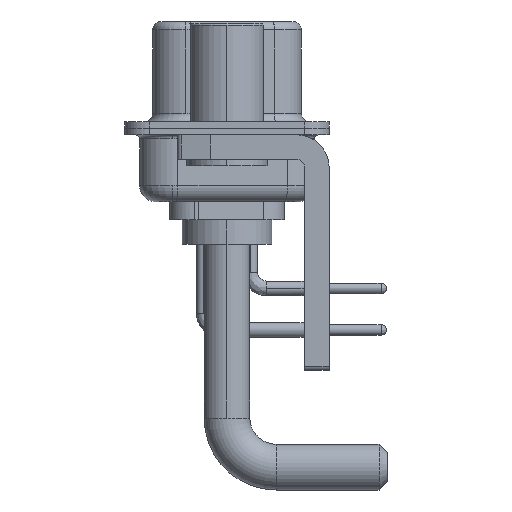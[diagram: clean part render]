
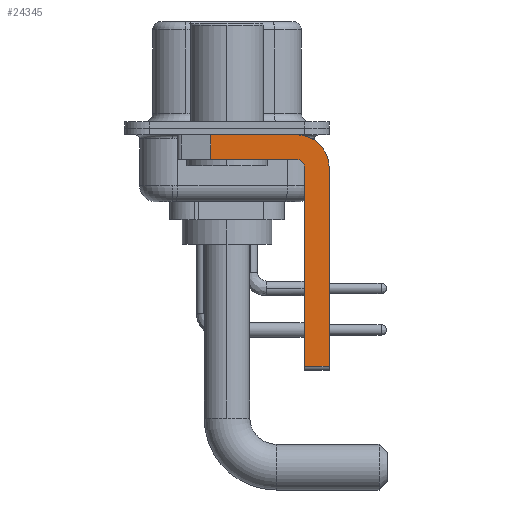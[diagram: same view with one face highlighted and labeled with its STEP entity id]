
A CAD part, left-side view. The second image highlights one B-rep face of the part: STEP entity #24345.
In plain terms, the highlighted planar face has unit normal (-1, 0, 0).
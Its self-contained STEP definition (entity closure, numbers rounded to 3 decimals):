
#410 = EDGE_CURVE ( 'NONE', #25710, #27441, #6920, .T. ) ;
#565 = DIRECTION ( 'NONE',  ( 0., -1., 0. ) ) ;
#676 = ORIENTED_EDGE ( 'NONE', *, *, #14166, .F. ) ;
#1849 = VERTEX_POINT ( 'NONE', #20379 ) ;
#2026 = ORIENTED_EDGE ( 'NONE', *, *, #20339, .F. ) ;
#2168 = EDGE_LOOP ( 'NONE', ( #2026, #29810, #25829, #3208, #10950, #25883, #17751, #676 ) ) ;
#2420 = AXIS2_PLACEMENT_3D ( 'NONE', #17290, #24402, #12674 ) ;
#2593 = CARTESIAN_POINT ( 'NONE',  ( -2.9, -4.75, -14.55 ) ) ;
#2806 = DIRECTION ( 'NONE',  ( 0., 0., 1. ) ) ;
#2974 = DIRECTION ( 'NONE',  ( -1., 0., 0. ) ) ;
#3181 = AXIS2_PLACEMENT_3D ( 'NONE', #6492, #15564, #27606 ) ;
#3208 = ORIENTED_EDGE ( 'NONE', *, *, #18490, .F. ) ;
#3356 = VECTOR ( 'NONE', #565, 1000. ) ;
#4076 = VECTOR ( 'NONE', #12142, 1000. ) ;
#4272 = CARTESIAN_POINT ( 'NONE',  ( -2.9, -4.25, -1.9 ) ) ;
#5451 = EDGE_CURVE ( 'NONE', #25708, #7545, #9273, .T. ) ;
#5493 = LINE ( 'NONE', #26307, #3356 ) ;
#5952 = CARTESIAN_POINT ( 'NONE',  ( -2.9, 3., -0.4 ) ) ;
#6468 = VECTOR ( 'NONE', #22313, 1000. ) ;
#6492 = CARTESIAN_POINT ( 'NONE',  ( -2.9, -4.25, -2.4 ) ) ;
#6920 = LINE ( 'NONE', #14143, #4076 ) ;
#7116 = CARTESIAN_POINT ( 'NONE',  ( -2.9, -4.75, -14.8 ) ) ;
#7545 = VERTEX_POINT ( 'NONE', #29081 ) ;
#7632 = EDGE_CURVE ( 'NONE', #21682, #27441, #29221, .T. ) ;
#8356 = LINE ( 'NONE', #8496, #16142 ) ;
#8496 = CARTESIAN_POINT ( 'NONE',  ( -2.9, -6.25, -2.4 ) ) ;
#9273 = LINE ( 'NONE', #7116, #28957 ) ;
#10350 = VERTEX_POINT ( 'NONE', #19581 ) ;
#10367 = CARTESIAN_POINT ( 'NONE',  ( -2.9, -4.25, -2.4 ) ) ;
#10745 = AXIS2_PLACEMENT_3D ( 'NONE', #10367, #2974, #2806 ) ;
#10950 = ORIENTED_EDGE ( 'NONE', *, *, #5451, .F. ) ;
#11106 = FACE_OUTER_BOUND ( 'NONE', #2168, .T. ) ;
#12142 = DIRECTION ( 'NONE',  ( 0., 1., 0. ) ) ;
#12674 = DIRECTION ( 'NONE',  ( 0., 0., -1. ) ) ;
#13794 = CARTESIAN_POINT ( 'NONE',  ( -2.9, 0.978, -1.9 ) ) ;
#14143 = CARTESIAN_POINT ( 'NONE',  ( -2.9, -4.25, -1.9 ) ) ;
#14166 = EDGE_CURVE ( 'NONE', #1849, #10350, #26072, .T. ) ;
#15564 = DIRECTION ( 'NONE',  ( 1., 0., 0. ) ) ;
#16142 = VECTOR ( 'NONE', #19890, 1000. ) ;
#16488 = DIRECTION ( 'NONE',  ( 0., 0., 1. ) ) ;
#16515 = CARTESIAN_POINT ( 'NONE',  ( -2.9, -6.25, -14.55 ) ) ;
#16962 = CARTESIAN_POINT ( 'NONE',  ( -2.9, 0.978, -0.4 ) ) ;
#17290 = CARTESIAN_POINT ( 'NONE',  ( -2.9, -4.25, -2.4 ) ) ;
#17751 = ORIENTED_EDGE ( 'NONE', *, *, #18556, .F. ) ;
#18490 = EDGE_CURVE ( 'NONE', #7545, #25710, #24050, .T. ) ;
#18556 = EDGE_CURVE ( 'NONE', #10350, #20711, #8356, .T. ) ;
#18698 = VECTOR ( 'NONE', #21825, 1000. ) ;
#19581 = CARTESIAN_POINT ( 'NONE',  ( -2.9, -6.25, -2.4 ) ) ;
#19890 = DIRECTION ( 'NONE',  ( 0., 0., -1. ) ) ;
#20339 = EDGE_CURVE ( 'NONE', #21682, #1849, #24897, .T. ) ;
#20379 = CARTESIAN_POINT ( 'NONE',  ( -2.9, -4.25, -0.4 ) ) ;
#20711 = VERTEX_POINT ( 'NONE', #16515 ) ;
#21682 = VERTEX_POINT ( 'NONE', #16962 ) ;
#21825 = DIRECTION ( 'NONE',  ( 0., -1., 0. ) ) ;
#22313 = DIRECTION ( 'NONE',  ( 0., 0., -1. ) ) ;
#24050 = CIRCLE ( 'NONE', #10745, 0.5 ) ;
#24345 = ADVANCED_FACE ( 'NONE', ( #11106 ), #29034, .F. ) ;
#24402 = DIRECTION ( 'NONE',  ( 1., 0., 0. ) ) ;
#24897 = LINE ( 'NONE', #5952, #18698 ) ;
#25708 = VERTEX_POINT ( 'NONE', #2593 ) ;
#25710 = VERTEX_POINT ( 'NONE', #4272 ) ;
#25829 = ORIENTED_EDGE ( 'NONE', *, *, #410, .F. ) ;
#25883 = ORIENTED_EDGE ( 'NONE', *, *, #29876, .T. ) ;
#26072 = CIRCLE ( 'NONE', #2420, 2. ) ;
#26307 = CARTESIAN_POINT ( 'NONE',  ( -2.9, -4.25, -14.55 ) ) ;
#27242 = CARTESIAN_POINT ( 'NONE',  ( -2.9, 0.978, -1.9 ) ) ;
#27441 = VERTEX_POINT ( 'NONE', #13794 ) ;
#27606 = DIRECTION ( 'NONE',  ( 0., 0., -1. ) ) ;
#28957 = VECTOR ( 'NONE', #16488, 1000. ) ;
#29034 = PLANE ( 'NONE',  #3181 ) ;
#29081 = CARTESIAN_POINT ( 'NONE',  ( -2.9, -4.75, -2.4 ) ) ;
#29221 = LINE ( 'NONE', #27242, #6468 ) ;
#29810 = ORIENTED_EDGE ( 'NONE', *, *, #7632, .T. ) ;
#29876 = EDGE_CURVE ( 'NONE', #25708, #20711, #5493, .T. ) ;
